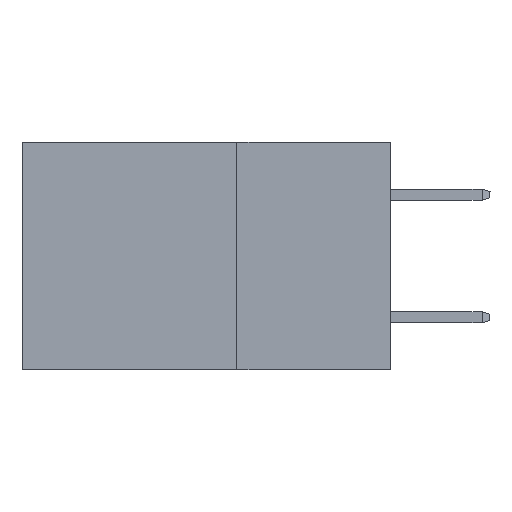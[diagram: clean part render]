
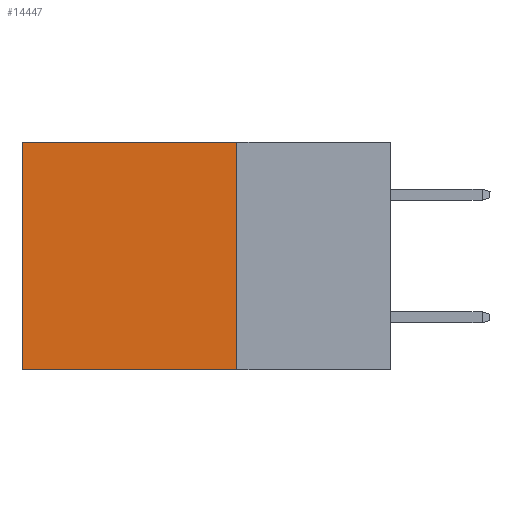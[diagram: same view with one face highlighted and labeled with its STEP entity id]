
A CAD part, left-side view. The second image highlights one B-rep face of the part: STEP entity #14447.
In plain terms, the highlighted planar face has unit normal (-1, 0, 0).
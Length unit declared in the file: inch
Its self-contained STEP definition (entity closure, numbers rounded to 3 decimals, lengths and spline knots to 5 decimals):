
#361 = ORIENTED_EDGE ( 'NONE', *, *, #16105, .T. ) ;
#1129 = DIRECTION ( 'NONE',  ( 0., 0., -1. ) ) ;
#1897 = CARTESIAN_POINT ( 'NONE',  ( 0.2875, 0.25, 0. ) ) ;
#2540 = ORIENTED_EDGE ( 'NONE', *, *, #13735, .F. ) ;
#2669 = CARTESIAN_POINT ( 'NONE',  ( 0.2875, 0.25, 0. ) ) ;
#3072 = VERTEX_POINT ( 'NONE', #14294 ) ;
#4388 = LINE ( 'NONE', #2669, #7430 ) ;
#4436 = PLANE ( 'NONE',  #10877 ) ;
#4778 = VERTEX_POINT ( 'NONE', #10467 ) ;
#4903 = EDGE_CURVE ( 'NONE', #4778, #5284, #7989, .T. ) ;
#5102 = CARTESIAN_POINT ( 'NONE',  ( 0.2875, 0.6, -0.37 ) ) ;
#5284 = VERTEX_POINT ( 'NONE', #5102 ) ;
#5765 = DIRECTION ( 'NONE',  ( 0., 0., -1. ) ) ;
#5843 = CARTESIAN_POINT ( 'NONE',  ( 0.2875, 0.25, -0.37 ) ) ;
#6068 = DIRECTION ( 'NONE',  ( 0., 1., 0. ) ) ;
#7085 = FACE_OUTER_BOUND ( 'NONE', #12310, .T. ) ;
#7430 = VECTOR ( 'NONE', #13985, 39.37008 ) ;
#7675 = VERTEX_POINT ( 'NONE', #5843 ) ;
#7989 = LINE ( 'NONE', #11941, #14167 ) ;
#8552 = ORIENTED_EDGE ( 'NONE', *, *, #4903, .T. ) ;
#9406 = VECTOR ( 'NONE', #1129, 39.37008 ) ;
#10467 = CARTESIAN_POINT ( 'NONE',  ( 0.2875, 0.6, 0. ) ) ;
#10877 = AXIS2_PLACEMENT_3D ( 'NONE', #1897, #13249, #5765 ) ;
#11281 = CARTESIAN_POINT ( 'NONE',  ( 0.2875, 0.25, 0. ) ) ;
#11436 = VECTOR ( 'NONE', #6068, 39.37008 ) ;
#11797 = LINE ( 'NONE', #15880, #11436 ) ;
#11941 = CARTESIAN_POINT ( 'NONE',  ( 0.2875, 0.6, 0. ) ) ;
#12310 = EDGE_LOOP ( 'NONE', ( #8552, #2540, #12643, #361 ) ) ;
#12643 = ORIENTED_EDGE ( 'NONE', *, *, #15954, .F. ) ;
#13176 = DIRECTION ( 'NONE',  ( 0., 0., -1. ) ) ;
#13249 = DIRECTION ( 'NONE',  ( 1., 0., 0. ) ) ;
#13440 = LINE ( 'NONE', #11281, #9406 ) ;
#13735 = EDGE_CURVE ( 'NONE', #7675, #5284, #11797, .T. ) ;
#13985 = DIRECTION ( 'NONE',  ( 0., 1., 0. ) ) ;
#14167 = VECTOR ( 'NONE', #13176, 39.37008 ) ;
#14294 = CARTESIAN_POINT ( 'NONE',  ( 0.2875, 0.25, 0. ) ) ;
#14447 = ADVANCED_FACE ( 'NONE', ( #7085 ), #4436, .F. ) ;
#15880 = CARTESIAN_POINT ( 'NONE',  ( 0.2875, 0.25, -0.37 ) ) ;
#15954 = EDGE_CURVE ( 'NONE', #3072, #7675, #13440, .T. ) ;
#16105 = EDGE_CURVE ( 'NONE', #3072, #4778, #4388, .T. ) ;
